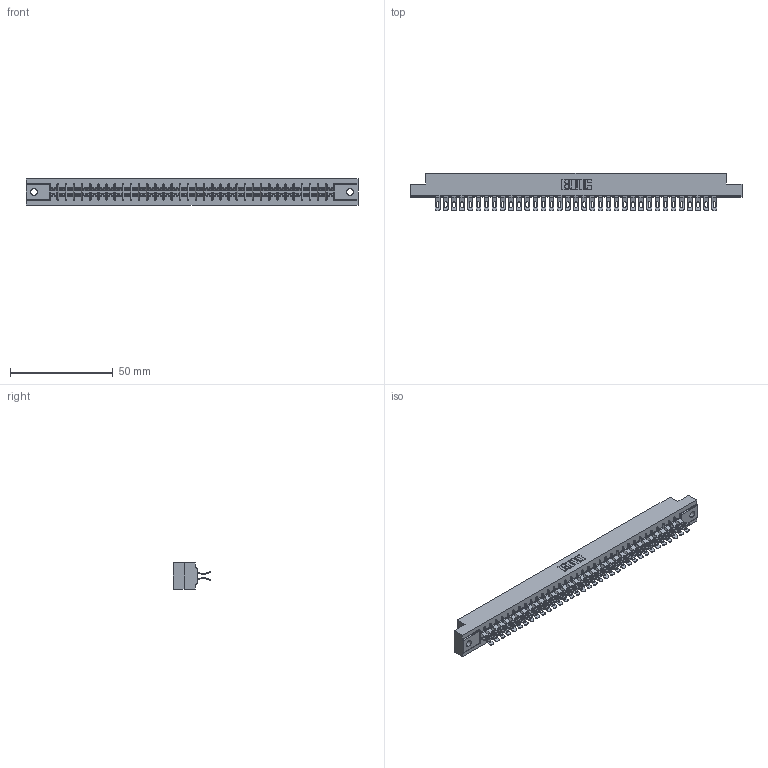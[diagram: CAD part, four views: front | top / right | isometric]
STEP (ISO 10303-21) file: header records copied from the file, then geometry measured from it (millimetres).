
FILE_DESCRIPTION (( 'STEP AP203' ), '1' );
FILE_NAME ('315-070-555-202.STEP', '2019-09-10T21:31:43', ( '' ), ( '' ), 'SwSTEP 2.0', 'SolidWorks 2016', '' );
FILE_SCHEMA (( 'CONFIG_CONTROL_DESIGN' ));
Length unit declared in the file: inch
Products named in the file (3): 305 Part_.128 Dia; 305-290-001_555; 315-070-555-202
Assembly tree (71 placements, depth 2):
  315-070-555-202
    305 Part_.128 Dia
    305-290-001_555  x70
Bounding box: 161.7 x 18.41 x 12.7 mm (x, y, z)
Volume: 16999.5 mm3; surface area: 22506.9 mm2
Topology: 71 solids, 71 shells, 4736 faces, 14141 edges, 9238 vertices
Faces by surface type: plane 2308, cylinder 2288, sphere 140
Entity records: 39374 total; most frequent: CARTESIAN_POINT 6533, ORIENTED_EDGE 6474, DIRECTION 6319, EDGE_CURVE 3237, LINE 2591, VECTOR 2591, VERTEX_POINT 2062, AXIS2_PLACEMENT_3D 1864
